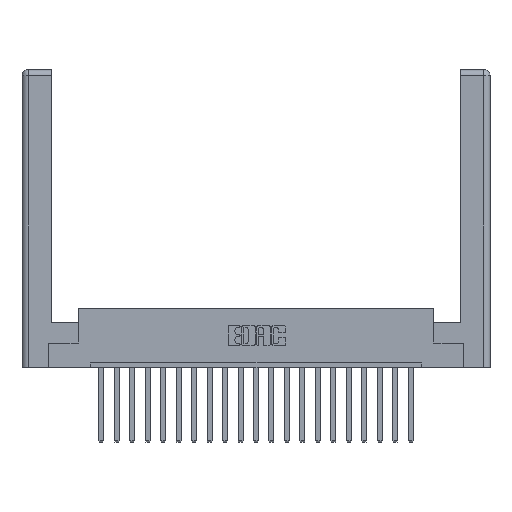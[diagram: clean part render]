
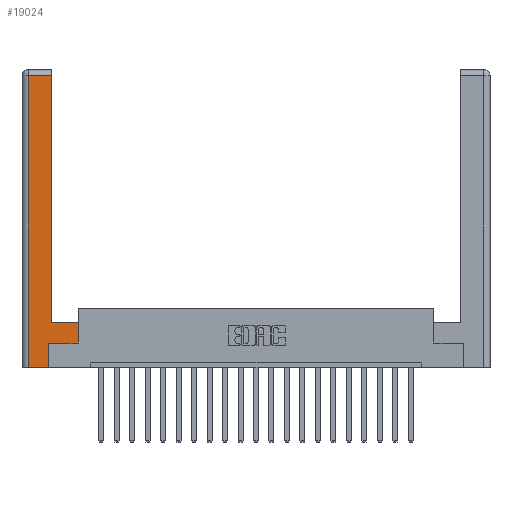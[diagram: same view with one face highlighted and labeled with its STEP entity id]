
A CAD part, top view. The second image highlights one B-rep face of the part: STEP entity #19024.
In plain terms, the highlighted planar face has unit normal (0, 0, 1).
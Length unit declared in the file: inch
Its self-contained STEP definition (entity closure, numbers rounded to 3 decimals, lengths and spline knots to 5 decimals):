
#41 = EDGE_CURVE ( 'NONE', #3376, #20408, #13714, .T. ) ;
#62 = CARTESIAN_POINT ( 'NONE',  ( 0.565, 0.245, 0. ) ) ;
#152 = VECTOR ( 'NONE', #4607, 39.37008 ) ;
#1492 = VECTOR ( 'NONE', #9258, 39.37008 ) ;
#1510 = CARTESIAN_POINT ( 'NONE',  ( 0.295, 3., 0. ) ) ;
#2346 = ORIENTED_EDGE ( 'NONE', *, *, #9121, .T. ) ;
#2563 = LINE ( 'NONE', #1510, #5605 ) ;
#2658 = DIRECTION ( 'NONE',  ( 0., 1., 0. ) ) ;
#3376 = VERTEX_POINT ( 'NONE', #5575 ) ;
#3490 = LINE ( 'NONE', #16537, #12003 ) ;
#3495 = CARTESIAN_POINT ( 'NONE',  ( 0.295, 0.45, 0. ) ) ;
#3899 = VECTOR ( 'NONE', #10779, 39.37008 ) ;
#3991 = ORIENTED_EDGE ( 'NONE', *, *, #4589, .T. ) ;
#4589 = EDGE_CURVE ( 'NONE', #17673, #16511, #10646, .T. ) ;
#4607 = DIRECTION ( 'NONE',  ( 1., 0., 0. ) ) ;
#4957 = DIRECTION ( 'NONE',  ( 0., 1., 0. ) ) ;
#5368 = DIRECTION ( 'NONE',  ( 1., 0., 0. ) ) ;
#5548 = DIRECTION ( 'NONE',  ( -1., 0., 0. ) ) ;
#5575 = CARTESIAN_POINT ( 'NONE',  ( 0.265, 0.245, 0. ) ) ;
#5605 = VECTOR ( 'NONE', #8290, 39.37008 ) ;
#6973 = VERTEX_POINT ( 'NONE', #9940 ) ;
#7211 = CARTESIAN_POINT ( 'NONE',  ( 0.0615, 0., 0. ) ) ;
#7245 = FACE_OUTER_BOUND ( 'NONE', #20133, .T. ) ;
#7639 = ORIENTED_EDGE ( 'NONE', *, *, #20103, .T. ) ;
#8290 = DIRECTION ( 'NONE',  ( 0., 1., 0. ) ) ;
#8834 = ORIENTED_EDGE ( 'NONE', *, *, #11634, .T. ) ;
#9121 = EDGE_CURVE ( 'NONE', #19614, #9396, #3490, .T. ) ;
#9258 = DIRECTION ( 'NONE',  ( 0., -1., 0. ) ) ;
#9396 = VERTEX_POINT ( 'NONE', #17932 ) ;
#9940 = CARTESIAN_POINT ( 'NONE',  ( 0.295, 2.94, 0. ) ) ;
#10532 = CARTESIAN_POINT ( 'NONE',  ( 0.0615, 2.94, 0. ) ) ;
#10646 = LINE ( 'NONE', #15441, #3899 ) ;
#10737 = DIRECTION ( 'NONE',  ( 0., 0., -1. ) ) ;
#10752 = LINE ( 'NONE', #15523, #14976 ) ;
#10779 = DIRECTION ( 'NONE',  ( -1., 0., 0. ) ) ;
#11084 = CARTESIAN_POINT ( 'NONE',  ( 0.565, 0.245, 0. ) ) ;
#11504 = VECTOR ( 'NONE', #5548, 39.37008 ) ;
#11634 = EDGE_CURVE ( 'NONE', #16511, #6973, #2563, .T. ) ;
#12003 = VECTOR ( 'NONE', #5368, 39.37008 ) ;
#12617 = DIRECTION ( 'NONE',  ( -1., 0., 0. ) ) ;
#12679 = ORIENTED_EDGE ( 'NONE', *, *, #14071, .T. ) ;
#12714 = EDGE_CURVE ( 'NONE', #20084, #19614, #18585, .T. ) ;
#13714 = LINE ( 'NONE', #62, #152 ) ;
#13911 = VECTOR ( 'NONE', #2658, 39.37008 ) ;
#14071 = EDGE_CURVE ( 'NONE', #20408, #17673, #10752, .T. ) ;
#14510 = EDGE_CURVE ( 'NONE', #6973, #20084, #19487, .T. ) ;
#14976 = VECTOR ( 'NONE', #4957, 39.37008 ) ;
#14981 = PLANE ( 'NONE',  #18669 ) ;
#15395 = CARTESIAN_POINT ( 'NONE',  ( 0., 0., 0. ) ) ;
#15441 = CARTESIAN_POINT ( 'NONE',  ( 0.295, 0.45, 0. ) ) ;
#15523 = CARTESIAN_POINT ( 'NONE',  ( 0.565, 0.45, 0. ) ) ;
#16141 = LINE ( 'NONE', #17079, #13911 ) ;
#16511 = VERTEX_POINT ( 'NONE', #3495 ) ;
#16537 = CARTESIAN_POINT ( 'NONE',  ( 0.265, 0., 0. ) ) ;
#16698 = ORIENTED_EDGE ( 'NONE', *, *, #12714, .T. ) ;
#16921 = ORIENTED_EDGE ( 'NONE', *, *, #41, .T. ) ;
#17079 = CARTESIAN_POINT ( 'NONE',  ( 0.265, 0.245, 0. ) ) ;
#17673 = VERTEX_POINT ( 'NONE', #18865 ) ;
#17682 = ORIENTED_EDGE ( 'NONE', *, *, #14510, .T. ) ;
#17932 = CARTESIAN_POINT ( 'NONE',  ( 0.265, 0., 0. ) ) ;
#18167 = CARTESIAN_POINT ( 'NONE',  ( 0.0615, 2.94, 0. ) ) ;
#18585 = LINE ( 'NONE', #20202, #1492 ) ;
#18669 = AXIS2_PLACEMENT_3D ( 'NONE', #15395, #10737, #12617 ) ;
#18865 = CARTESIAN_POINT ( 'NONE',  ( 0.565, 0.45, 0. ) ) ;
#19024 = ADVANCED_FACE ( 'NONE', ( #7245 ), #14981, .F. ) ;
#19487 = LINE ( 'NONE', #10532, #11504 ) ;
#19614 = VERTEX_POINT ( 'NONE', #7211 ) ;
#20084 = VERTEX_POINT ( 'NONE', #18167 ) ;
#20103 = EDGE_CURVE ( 'NONE', #9396, #3376, #16141, .T. ) ;
#20133 = EDGE_LOOP ( 'NONE', ( #8834, #17682, #16698, #2346, #7639, #16921, #12679, #3991 ) ) ;
#20202 = CARTESIAN_POINT ( 'NONE',  ( 0.0615, 0., 0. ) ) ;
#20408 = VERTEX_POINT ( 'NONE', #11084 ) ;
